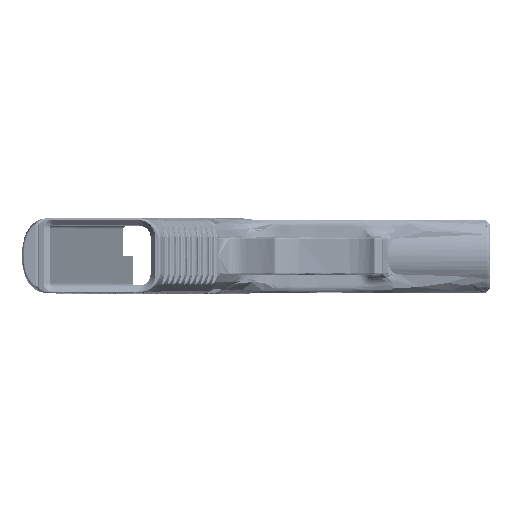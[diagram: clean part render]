
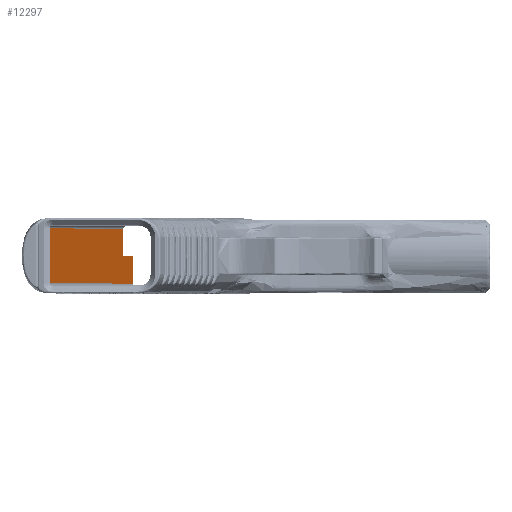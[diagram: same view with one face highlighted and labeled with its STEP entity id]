
A CAD part, top view. The second image highlights one B-rep face of the part: STEP entity #12297.
In plain terms, the highlighted planar face has unit normal (0.951, 0, 0.309).
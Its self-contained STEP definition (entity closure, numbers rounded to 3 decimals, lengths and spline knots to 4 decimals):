
#8022 = EDGE_CURVE ( 'NONE', #370960, #202831, #40710, .T. ) ;
#12297 = ADVANCED_FACE ( 'NONE', ( #225261 ), #376204, .F. ) ;
#34640 = VECTOR ( 'NONE', #217632, 39.3701 ) ;
#37832 = CARTESIAN_POINT ( 'NONE',  ( 1.9466, 0.37, -3.4826 ) ) ;
#40710 = LINE ( 'NONE', #325596, #276852 ) ;
#54026 = CARTESIAN_POINT ( 'NONE',  ( 1.9466, 0., -3.4826 ) ) ;
#61543 = VERTEX_POINT ( 'NONE', #229214 ) ;
#71822 = CARTESIAN_POINT ( 'NONE',  ( 2.0809, 0., -3.896 ) ) ;
#79664 = VECTOR ( 'NONE', #257630, 39.3701 ) ;
#98699 = DIRECTION ( 'NONE',  ( -0.309, 0., 0.951 ) ) ;
#109622 = AXIS2_PLACEMENT_3D ( 'NONE', #190170, #130879, #98699 ) ;
#128240 = DIRECTION ( 'NONE',  ( 0., 1., 0. ) ) ;
#130879 = DIRECTION ( 'NONE',  ( -0.951, 0., -0.309 ) ) ;
#132387 = EDGE_CURVE ( 'NONE', #202831, #385903, #197264, .T. ) ;
#147120 = LINE ( 'NONE', #71822, #79664 ) ;
#149459 = ORIENTED_EDGE ( 'NONE', *, *, #8022, .F. ) ;
#151765 = CARTESIAN_POINT ( 'NONE',  ( 2.0809, -0.37, -3.896 ) ) ;
#156533 = CARTESIAN_POINT ( 'NONE',  ( 0.9499, 0., -0.4151 ) ) ;
#165273 = CARTESIAN_POINT ( 'NONE',  ( 0.9499, 0.37, -0.4151 ) ) ;
#168166 = ORIENTED_EDGE ( 'NONE', *, *, #305519, .F. ) ;
#181104 = VERTEX_POINT ( 'NONE', #210322 ) ;
#183390 = CARTESIAN_POINT ( 'NONE',  ( 1.9466, 0.0001, -3.4826 ) ) ;
#190170 = CARTESIAN_POINT ( 'NONE',  ( 2.0746, 0., -3.8765 ) ) ;
#197264 = LINE ( 'NONE', #54026, #390305 ) ;
#198498 = ORIENTED_EDGE ( 'NONE', *, *, #224967, .F. ) ;
#201905 = VECTOR ( 'NONE', #128240, 39.3701 ) ;
#202831 = VERTEX_POINT ( 'NONE', #37832 ) ;
#205956 = LINE ( 'NONE', #254729, #248861 ) ;
#210322 = CARTESIAN_POINT ( 'NONE',  ( 2.0809, 0.0001, -3.896 ) ) ;
#217632 = DIRECTION ( 'NONE',  ( 0.309, 0., -0.951 ) ) ;
#218961 = CARTESIAN_POINT ( 'NONE',  ( 2.0746, 0.0001, -3.8765 ) ) ;
#221012 = DIRECTION ( 'NONE',  ( -0.309, 0., 0.951 ) ) ;
#224967 = EDGE_CURVE ( 'NONE', #385903, #181104, #381728, .T. ) ;
#225261 = FACE_OUTER_BOUND ( 'NONE', #287902, .T. ) ;
#229214 = CARTESIAN_POINT ( 'NONE',  ( 0.9499, -0.37, -0.4151 ) ) ;
#232581 = DIRECTION ( 'NONE',  ( 0.309, 0., -0.951 ) ) ;
#241135 = DIRECTION ( 'NONE',  ( 0., -1., 0. ) ) ;
#245294 = EDGE_CURVE ( 'NONE', #181104, #320419, #147120, .T. ) ;
#248861 = VECTOR ( 'NONE', #221012, 39.3701 ) ;
#254729 = CARTESIAN_POINT ( 'NONE',  ( 2.0746, -0.37, -3.8765 ) ) ;
#257362 = EDGE_CURVE ( 'NONE', #320419, #61543, #205956, .T. ) ;
#257630 = DIRECTION ( 'NONE',  ( 0., -1., 0. ) ) ;
#275753 = ORIENTED_EDGE ( 'NONE', *, *, #245294, .F. ) ;
#276852 = VECTOR ( 'NONE', #232581, 39.3701 ) ;
#287902 = EDGE_LOOP ( 'NONE', ( #376300, #149459, #168166, #398628, #275753, #198498 ) ) ;
#305519 = EDGE_CURVE ( 'NONE', #61543, #370960, #312930, .T. ) ;
#312930 = LINE ( 'NONE', #156533, #201905 ) ;
#320419 = VERTEX_POINT ( 'NONE', #151765 ) ;
#325596 = CARTESIAN_POINT ( 'NONE',  ( 2.0746, 0.37, -3.8765 ) ) ;
#370960 = VERTEX_POINT ( 'NONE', #165273 ) ;
#376204 = PLANE ( 'NONE',  #109622 ) ;
#376300 = ORIENTED_EDGE ( 'NONE', *, *, #132387, .F. ) ;
#381728 = LINE ( 'NONE', #218961, #34640 ) ;
#385903 = VERTEX_POINT ( 'NONE', #183390 ) ;
#390305 = VECTOR ( 'NONE', #241135, 39.3701 ) ;
#398628 = ORIENTED_EDGE ( 'NONE', *, *, #257362, .F. ) ;
